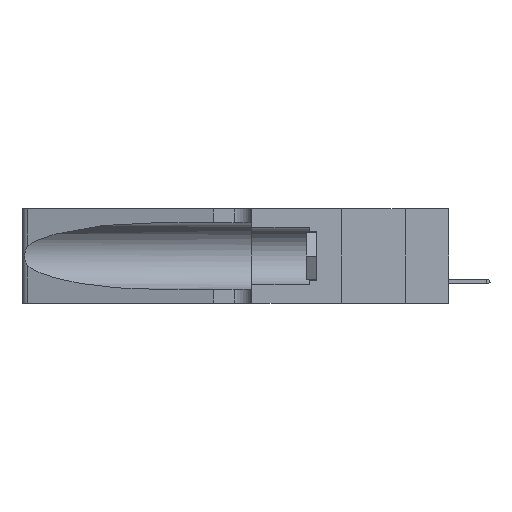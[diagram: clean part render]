
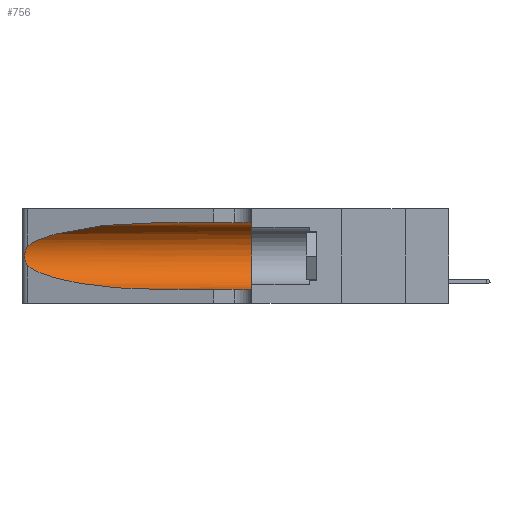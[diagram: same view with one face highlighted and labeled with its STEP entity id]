
A CAD part, left-side view. The second image highlights one B-rep face of the part: STEP entity #756.
In plain terms, the highlighted cylindrical face has radius 3.308 mm (diameter 6.617 mm), a partial arc.
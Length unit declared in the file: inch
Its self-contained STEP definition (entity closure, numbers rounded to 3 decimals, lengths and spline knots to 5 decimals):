
#756 = ADVANCED_FACE ( 'NONE', ( #12771 ), #27107, .F. ) ;
#1384 = CARTESIAN_POINT ( 'NONE',  ( 0.25487, 1.22718, 0.22369 ) ) ;
#1541 = EDGE_CURVE ( 'NONE', #30630, #13859, #3413, .T. ) ;
#1738 = DIRECTION ( 'NONE',  ( 0., -1., 0. ) ) ;
#2438 = CARTESIAN_POINT ( 'NONE',  ( 0.1305, 0.35, 0.185 ) ) ;
#3413 =( BOUNDED_CURVE ( )  B_SPLINE_CURVE ( 3, ( #19828, #12567, #7876, #29888 ),
 .UNSPECIFIED., .F., .T. ) 
 B_SPLINE_CURVE_WITH_KNOTS ( ( 4, 4 ),
 ( 3.44316, 4.71239 ),
 .UNSPECIFIED. ) 
 CURVE ( )  GEOMETRIC_REPRESENTATION_ITEM ( )  RATIONAL_B_SPLINE_CURVE ( ( 1., 0.87, 0.87, 1. ) ) 
 REPRESENTATION_ITEM ( '' )  );
#3436 = ORIENTED_EDGE ( 'NONE', *, *, #1541, .T. ) ;
#3630 = CARTESIAN_POINT ( 'NONE',  ( 0.25789, 1.23486, 0.15765 ) ) ;
#3747 = CARTESIAN_POINT ( 'NONE',  ( 0.25639, 1.23184, 0.21858 ) ) ;
#3864 = CARTESIAN_POINT ( 'NONE',  ( 0.26075, 1.23896, 0.178 ) ) ;
#4006 = DIRECTION ( 'NONE',  ( 0., 0., -1. ) ) ;
#4139 = CARTESIAN_POINT ( 'NONE',  ( 0.1305, 0.35, 0.31525 ) ) ;
#4279 = LINE ( 'NONE', #13963, #16669 ) ;
#4802 = DIRECTION ( 'NONE',  ( 0., -1., 0. ) ) ;
#5184 = LINE ( 'NONE', #19525, #19159 ) ;
#6015 = CARTESIAN_POINT ( 'NONE',  ( 0.18966, 0.96281, 0.31525 ) ) ;
#6269 = CARTESIAN_POINT ( 'NONE',  ( 0.25555, 1.22994, 0.2215 ) ) ;
#6384 = CARTESIAN_POINT ( 'NONE',  ( 0.25856, 1.23593, 0.16098 ) ) ;
#7876 = CARTESIAN_POINT ( 'NONE',  ( 0.18966, 0.96281, 0.05475 ) ) ;
#8635 = CARTESIAN_POINT ( 'NONE',  ( 0.26075, 1.23896, 0.19203 ) ) ;
#9553 = CIRCLE ( 'NONE', #22510, 0.13025 ) ;
#9934 = DIRECTION ( 'NONE',  ( 0., 0., 1. ) ) ;
#10991 = CARTESIAN_POINT ( 'NONE',  ( 0.1305, 0.72297, 0.31525 ) ) ;
#11249 = CARTESIAN_POINT ( 'NONE',  ( 0.25787, 1.23484, 0.2124 ) ) ;
#11320 = VERTEX_POINT ( 'NONE', #18845 ) ;
#12497 = EDGE_CURVE ( 'NONE', #15905, #25498, #30245, .T. ) ;
#12567 = CARTESIAN_POINT ( 'NONE',  ( 0.2373, 1.15595, 0.08982 ) ) ;
#12771 = FACE_OUTER_BOUND ( 'NONE', #22302, .T. ) ;
#12908 = ORIENTED_EDGE ( 'NONE', *, *, #27925, .F. ) ;
#13539 = CARTESIAN_POINT ( 'NONE',  ( 0.25639, 1.23186, 0.15144 ) ) ;
#13859 = VERTEX_POINT ( 'NONE', #23091 ) ;
#13963 = CARTESIAN_POINT ( 'NONE',  ( 0.1305, 1.61858, 0.31525 ) ) ;
#14418 = VERTEX_POINT ( 'NONE', #4139 ) ;
#15171 = CARTESIAN_POINT ( 'NONE',  ( 0.25487, 1.22718, 0.14631 ) ) ;
#15905 = VERTEX_POINT ( 'NONE', #28193 ) ;
#16669 = VECTOR ( 'NONE', #26503, 39.37008 ) ;
#18259 = ORIENTED_EDGE ( 'NONE', *, *, #19489, .T. ) ;
#18374 = CARTESIAN_POINT ( 'NONE',  ( 0.26018, 1.23835, 0.19895 ) ) ;
#18712 = CARTESIAN_POINT ( 'NONE',  ( 0.25854, 1.2359, 0.20912 ) ) ;
#18845 = CARTESIAN_POINT ( 'NONE',  ( 0.1305, 0.35, 0.05475 ) ) ;
#19078 = CARTESIAN_POINT ( 'NONE',  ( 0.1305, 1.61858, 0.185 ) ) ;
#19159 = VECTOR ( 'NONE', #4802, 39.37008 ) ;
#19489 = EDGE_CURVE ( 'NONE', #25498, #30630, #22179, .T. ) ;
#19525 = CARTESIAN_POINT ( 'NONE',  ( 0.1305, 1.61858, 0.05475 ) ) ;
#19538 = AXIS2_PLACEMENT_3D ( 'NONE', #19078, #1738, #4006 ) ;
#19828 = CARTESIAN_POINT ( 'NONE',  ( 0.25487, 1.22718, 0.14631 ) ) ;
#21238 = CARTESIAN_POINT ( 'NONE',  ( 0.26017, 1.23833, 0.17102 ) ) ;
#22179 = B_SPLINE_CURVE_WITH_KNOTS ( 'NONE', 3,
 ( #1384, #6269, #3747, #11249, #18712, #18374, #8635, #3864, #21238, #6384, #3630, #13539, #23745, #25649 ),
 .UNSPECIFIED., .F., .F.,
 ( 4, 2, 2, 2, 2, 2, 4 ),
 ( 0., 0.00027, 0.00053, 0.00107, 0.0016, 0.00187, 0.00214 ),
 .UNSPECIFIED. ) ;
#22302 = EDGE_LOOP ( 'NONE', ( #26864, #18259, #3436, #23912, #12908, #30503 ) ) ;
#22510 = AXIS2_PLACEMENT_3D ( 'NONE', #2438, #27445, #9934 ) ;
#23091 = CARTESIAN_POINT ( 'NONE',  ( 0.1305, 0.72297, 0.05475 ) ) ;
#23260 = CARTESIAN_POINT ( 'NONE',  ( 0.2373, 1.15595, 0.28018 ) ) ;
#23745 = CARTESIAN_POINT ( 'NONE',  ( 0.25555, 1.22993, 0.14849 ) ) ;
#23912 = ORIENTED_EDGE ( 'NONE', *, *, #29267, .T. ) ;
#24935 = CARTESIAN_POINT ( 'NONE',  ( 0.25487, 1.22718, 0.22369 ) ) ;
#25498 = VERTEX_POINT ( 'NONE', #24935 ) ;
#25649 = CARTESIAN_POINT ( 'NONE',  ( 0.25487, 1.22718, 0.14631 ) ) ;
#26503 = DIRECTION ( 'NONE',  ( 0., -1., 0. ) ) ;
#26505 = EDGE_CURVE ( 'NONE', #15905, #14418, #4279, .T. ) ;
#26864 = ORIENTED_EDGE ( 'NONE', *, *, #12497, .T. ) ;
#27107 = CYLINDRICAL_SURFACE ( 'NONE', #19538, 0.13025 ) ;
#27445 = DIRECTION ( 'NONE',  ( 0., 1., 0. ) ) ;
#27925 = EDGE_CURVE ( 'NONE', #14418, #11320, #9553, .T. ) ;
#28193 = CARTESIAN_POINT ( 'NONE',  ( 0.1305, 0.72297, 0.31525 ) ) ;
#28532 = CARTESIAN_POINT ( 'NONE',  ( 0.25487, 1.22718, 0.22369 ) ) ;
#29267 = EDGE_CURVE ( 'NONE', #13859, #11320, #5184, .T. ) ;
#29888 = CARTESIAN_POINT ( 'NONE',  ( 0.1305, 0.72297, 0.05475 ) ) ;
#30245 =( BOUNDED_CURVE ( )  B_SPLINE_CURVE ( 3, ( #10991, #6015, #23260, #28532 ),
 .UNSPECIFIED., .F., .F. ) 
 B_SPLINE_CURVE_WITH_KNOTS ( ( 4, 4 ),
 ( 1.5708, 2.84003 ),
 .UNSPECIFIED. ) 
 CURVE ( )  GEOMETRIC_REPRESENTATION_ITEM ( )  RATIONAL_B_SPLINE_CURVE ( ( 1., 0.87, 0.87, 1. ) ) 
 REPRESENTATION_ITEM ( '' )  );
#30503 = ORIENTED_EDGE ( 'NONE', *, *, #26505, .F. ) ;
#30630 = VERTEX_POINT ( 'NONE', #15171 ) ;
